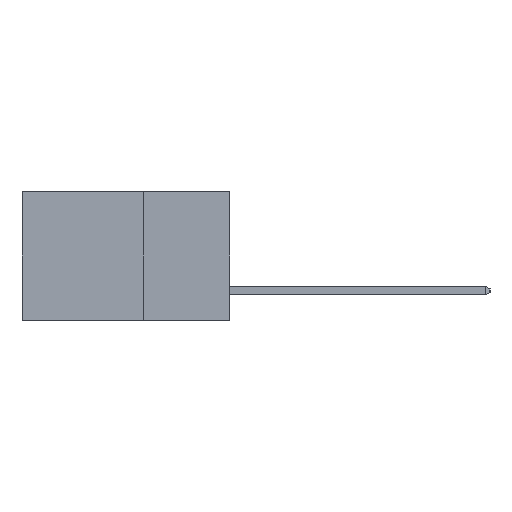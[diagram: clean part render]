
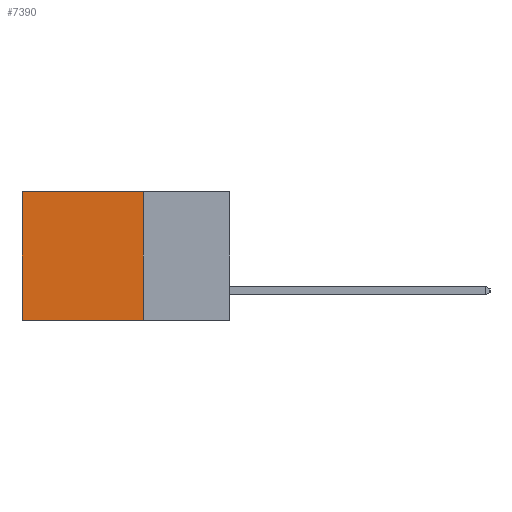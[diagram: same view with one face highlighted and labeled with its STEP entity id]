
A CAD part, left-side view. The second image highlights one B-rep face of the part: STEP entity #7390.
In plain terms, the highlighted planar face has unit normal (-1, 0, 0).
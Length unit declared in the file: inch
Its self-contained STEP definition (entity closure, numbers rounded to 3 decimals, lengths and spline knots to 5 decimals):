
#201 = EDGE_CURVE ( 'NONE', #11362, #10778, #9447, .T. ) ;
#1385 = VECTOR ( 'NONE', #5194, 39.37008 ) ;
#1597 = CARTESIAN_POINT ( 'NONE',  ( 0.298, 0.25, -0.37 ) ) ;
#1732 = LINE ( 'NONE', #4157, #7495 ) ;
#2197 = CARTESIAN_POINT ( 'NONE',  ( 0.298, 0.25, 0. ) ) ;
#2891 = PLANE ( 'NONE',  #5201 ) ;
#3043 = EDGE_LOOP ( 'NONE', ( #12256, #11998, #9309, #5954 ) ) ;
#3086 = CARTESIAN_POINT ( 'NONE',  ( 0.298, 0.6, 0. ) ) ;
#3775 = CARTESIAN_POINT ( 'NONE',  ( 0.298, 0.6, 0. ) ) ;
#4100 = FACE_OUTER_BOUND ( 'NONE', #3043, .T. ) ;
#4157 = CARTESIAN_POINT ( 'NONE',  ( 0.298, 0.25, 0. ) ) ;
#4452 = LINE ( 'NONE', #3775, #10116 ) ;
#5116 = CARTESIAN_POINT ( 'NONE',  ( 0.298, 0.25, -0.37 ) ) ;
#5194 = DIRECTION ( 'NONE',  ( 0., 1., 0. ) ) ;
#5201 = AXIS2_PLACEMENT_3D ( 'NONE', #5214, #13096, #6362 ) ;
#5214 = CARTESIAN_POINT ( 'NONE',  ( 0.298, 0.25, 0. ) ) ;
#5286 = DIRECTION ( 'NONE',  ( 0., 0., -1. ) ) ;
#5954 = ORIENTED_EDGE ( 'NONE', *, *, #11668, .T. ) ;
#6345 = CARTESIAN_POINT ( 'NONE',  ( 0.298, 0.6, -0.37 ) ) ;
#6362 = DIRECTION ( 'NONE',  ( 0., 0., -1. ) ) ;
#7390 = ADVANCED_FACE ( 'NONE', ( #4100 ), #2891, .F. ) ;
#7495 = VECTOR ( 'NONE', #5286, 39.37008 ) ;
#7926 = CARTESIAN_POINT ( 'NONE',  ( 0.298, 0.25, 0. ) ) ;
#8297 = VERTEX_POINT ( 'NONE', #7926 ) ;
#9039 = DIRECTION ( 'NONE',  ( 0., 1., 0. ) ) ;
#9309 = ORIENTED_EDGE ( 'NONE', *, *, #10823, .F. ) ;
#9447 = LINE ( 'NONE', #5116, #1385 ) ;
#10116 = VECTOR ( 'NONE', #12814, 39.37008 ) ;
#10778 = VERTEX_POINT ( 'NONE', #6345 ) ;
#10823 = EDGE_CURVE ( 'NONE', #8297, #11362, #1732, .T. ) ;
#11362 = VERTEX_POINT ( 'NONE', #1597 ) ;
#11668 = EDGE_CURVE ( 'NONE', #8297, #14440, #14608, .T. ) ;
#11717 = VECTOR ( 'NONE', #9039, 39.37008 ) ;
#11885 = EDGE_CURVE ( 'NONE', #14440, #10778, #4452, .T. ) ;
#11998 = ORIENTED_EDGE ( 'NONE', *, *, #201, .F. ) ;
#12256 = ORIENTED_EDGE ( 'NONE', *, *, #11885, .T. ) ;
#12814 = DIRECTION ( 'NONE',  ( 0., 0., -1. ) ) ;
#13096 = DIRECTION ( 'NONE',  ( 1., 0., 0. ) ) ;
#14440 = VERTEX_POINT ( 'NONE', #3086 ) ;
#14608 = LINE ( 'NONE', #2197, #11717 ) ;
